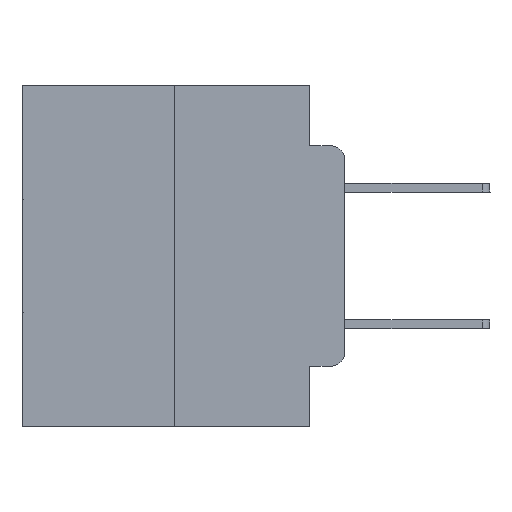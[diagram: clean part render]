
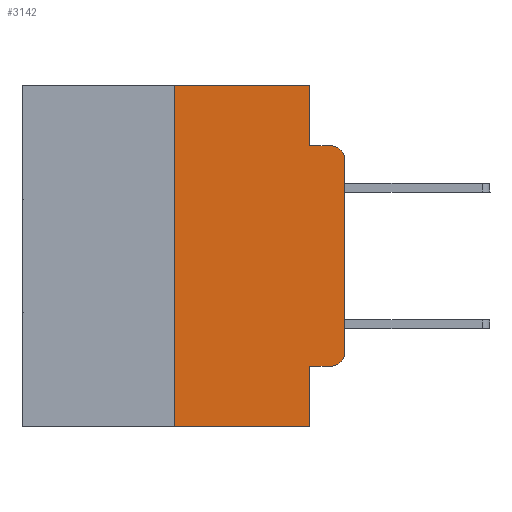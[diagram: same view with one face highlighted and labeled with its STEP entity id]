
A CAD part, left-side view. The second image highlights one B-rep face of the part: STEP entity #3142.
In plain terms, the highlighted planar face has unit normal (-1, 0, 0).
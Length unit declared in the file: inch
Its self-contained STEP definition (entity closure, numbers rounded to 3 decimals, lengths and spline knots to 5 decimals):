
#291 = LINE ( 'NONE', #4115, #11041 ) ;
#705 = DIRECTION ( 'NONE',  ( 0., 0., -1. ) ) ;
#1006 = EDGE_CURVE ( 'NONE', #3148, #11943, #18974, .T. ) ;
#1355 = VERTEX_POINT ( 'NONE', #27461 ) ;
#1722 = CARTESIAN_POINT ( 'NONE',  ( 0., 0.25, 0. ) ) ;
#2042 = LINE ( 'NONE', #16992, #23258 ) ;
#2127 = EDGE_CURVE ( 'NONE', #25146, #15685, #13877, .T. ) ;
#2295 = CARTESIAN_POINT ( 'NONE',  ( 0., 0.051, -0.5 ) ) ;
#3142 = ADVANCED_FACE ( 'NONE', ( #25592 ), #12815, .F. ) ;
#3148 = VERTEX_POINT ( 'NONE', #15057 ) ;
#3206 = LINE ( 'NONE', #3627, #11196 ) ;
#3627 = CARTESIAN_POINT ( 'NONE',  ( 0., 0.051, 0. ) ) ;
#4115 = CARTESIAN_POINT ( 'NONE',  ( 0., 0.051, -0.4115 ) ) ;
#4229 = CARTESIAN_POINT ( 'NONE',  ( 0., 0.473, 0. ) ) ;
#4906 = LINE ( 'NONE', #17885, #20362 ) ;
#5095 = CARTESIAN_POINT ( 'NONE',  ( 0., 0.25, 0. ) ) ;
#5928 = EDGE_CURVE ( 'NONE', #13244, #3148, #11708, .T. ) ;
#6202 = ORIENTED_EDGE ( 'NONE', *, *, #5928, .T. ) ;
#6298 = ORIENTED_EDGE ( 'NONE', *, *, #1006, .T. ) ;
#6406 = DIRECTION ( 'NONE',  ( 0., 0., 1. ) ) ;
#6814 = VECTOR ( 'NONE', #16111, 39.37008 ) ;
#6887 = AXIS2_PLACEMENT_3D ( 'NONE', #4229, #10673, #8980 ) ;
#7203 = VERTEX_POINT ( 'NONE', #9386 ) ;
#7260 = DIRECTION ( 'NONE',  ( 0., 0., -1. ) ) ;
#7308 = EDGE_CURVE ( 'NONE', #7203, #15796, #3206, .T. ) ;
#7484 = LINE ( 'NONE', #5095, #6814 ) ;
#8149 = DIRECTION ( 'NONE',  ( 0., -1., 0. ) ) ;
#8413 = ORIENTED_EDGE ( 'NONE', *, *, #26679, .F. ) ;
#8419 = ORIENTED_EDGE ( 'NONE', *, *, #20829, .F. ) ;
#8980 = DIRECTION ( 'NONE',  ( 0., 0., -1. ) ) ;
#9386 = CARTESIAN_POINT ( 'NONE',  ( 0., 0.051, 0. ) ) ;
#9889 = LINE ( 'NONE', #14559, #14706 ) ;
#10542 = EDGE_CURVE ( 'NONE', #1355, #15685, #4906, .T. ) ;
#10673 = DIRECTION ( 'NONE',  ( 1., 0., 0. ) ) ;
#10912 = EDGE_CURVE ( 'NONE', #11943, #26504, #20821, .T. ) ;
#11041 = VECTOR ( 'NONE', #23651, 39.37008 ) ;
#11196 = VECTOR ( 'NONE', #27398, 39.37008 ) ;
#11204 = DIRECTION ( 'NONE',  ( -1., 0., 0. ) ) ;
#11363 = ORIENTED_EDGE ( 'NONE', *, *, #2127, .F. ) ;
#11457 = ORIENTED_EDGE ( 'NONE', *, *, #10542, .T. ) ;
#11691 = CARTESIAN_POINT ( 'NONE',  ( 0., 0.051, -0.0885 ) ) ;
#11708 = CIRCLE ( 'NONE', #19393, 0.02 ) ;
#11738 = CARTESIAN_POINT ( 'NONE',  ( 0., 0.051, 0. ) ) ;
#11943 = VERTEX_POINT ( 'NONE', #20710 ) ;
#12815 = PLANE ( 'NONE',  #6887 ) ;
#13244 = VERTEX_POINT ( 'NONE', #13674 ) ;
#13674 = CARTESIAN_POINT ( 'NONE',  ( 0., 0.02, -0.4115 ) ) ;
#13877 = LINE ( 'NONE', #11738, #18038 ) ;
#14261 = VECTOR ( 'NONE', #6406, 39.37008 ) ;
#14559 = CARTESIAN_POINT ( 'NONE',  ( 0., 0.051, -0.0885 ) ) ;
#14706 = VECTOR ( 'NONE', #20615, 39.37008 ) ;
#15057 = CARTESIAN_POINT ( 'NONE',  ( 0., 0., -0.3915 ) ) ;
#15293 = CARTESIAN_POINT ( 'NONE',  ( 0., 0.051, -0.4115 ) ) ;
#15575 = DIRECTION ( 'NONE',  ( 0., 0., -1. ) ) ;
#15685 = VERTEX_POINT ( 'NONE', #2295 ) ;
#15796 = VERTEX_POINT ( 'NONE', #11691 ) ;
#16016 = ORIENTED_EDGE ( 'NONE', *, *, #26018, .T. ) ;
#16069 = CARTESIAN_POINT ( 'NONE',  ( 0., 0.02, -0.3915 ) ) ;
#16111 = DIRECTION ( 'NONE',  ( 0., 0., 1. ) ) ;
#16152 = ORIENTED_EDGE ( 'NONE', *, *, #27619, .F. ) ;
#16855 = DIRECTION ( 'NONE',  ( 0., -1., 0. ) ) ;
#16992 = CARTESIAN_POINT ( 'NONE',  ( 0., 0.473, 0. ) ) ;
#17885 = CARTESIAN_POINT ( 'NONE',  ( 0., 0.473, -0.5 ) ) ;
#18038 = VECTOR ( 'NONE', #15575, 39.37008 ) ;
#18282 = EDGE_LOOP ( 'NONE', ( #6298, #24316, #8413, #27099, #16152, #8419, #11457, #11363, #16016, #6202 ) ) ;
#18974 = LINE ( 'NONE', #23165, #14261 ) ;
#19393 = AXIS2_PLACEMENT_3D ( 'NONE', #16069, #24627, #705 ) ;
#19956 = CARTESIAN_POINT ( 'NONE',  ( 0., 0.02, -0.1085 ) ) ;
#20362 = VECTOR ( 'NONE', #8149, 39.37008 ) ;
#20615 = DIRECTION ( 'NONE',  ( 0., -1., 0. ) ) ;
#20710 = CARTESIAN_POINT ( 'NONE',  ( 0., 0., -0.1085 ) ) ;
#20821 = CIRCLE ( 'NONE', #22601, 0.02 ) ;
#20829 = EDGE_CURVE ( 'NONE', #1355, #24173, #7484, .T. ) ;
#22601 = AXIS2_PLACEMENT_3D ( 'NONE', #19956, #11204, #7260 ) ;
#23165 = CARTESIAN_POINT ( 'NONE',  ( 0., 0., 0. ) ) ;
#23258 = VECTOR ( 'NONE', #16855, 39.37008 ) ;
#23651 = DIRECTION ( 'NONE',  ( 0., -1., 0. ) ) ;
#24173 = VERTEX_POINT ( 'NONE', #1722 ) ;
#24316 = ORIENTED_EDGE ( 'NONE', *, *, #10912, .T. ) ;
#24627 = DIRECTION ( 'NONE',  ( -1., 0., 0. ) ) ;
#25146 = VERTEX_POINT ( 'NONE', #15293 ) ;
#25592 = FACE_OUTER_BOUND ( 'NONE', #18282, .T. ) ;
#26018 = EDGE_CURVE ( 'NONE', #25146, #13244, #291, .T. ) ;
#26473 = CARTESIAN_POINT ( 'NONE',  ( 0., 0.02, -0.0885 ) ) ;
#26504 = VERTEX_POINT ( 'NONE', #26473 ) ;
#26679 = EDGE_CURVE ( 'NONE', #15796, #26504, #9889, .T. ) ;
#27099 = ORIENTED_EDGE ( 'NONE', *, *, #7308, .F. ) ;
#27398 = DIRECTION ( 'NONE',  ( 0., 0., -1. ) ) ;
#27461 = CARTESIAN_POINT ( 'NONE',  ( 0., 0.25, -0.5 ) ) ;
#27619 = EDGE_CURVE ( 'NONE', #24173, #7203, #2042, .T. ) ;
